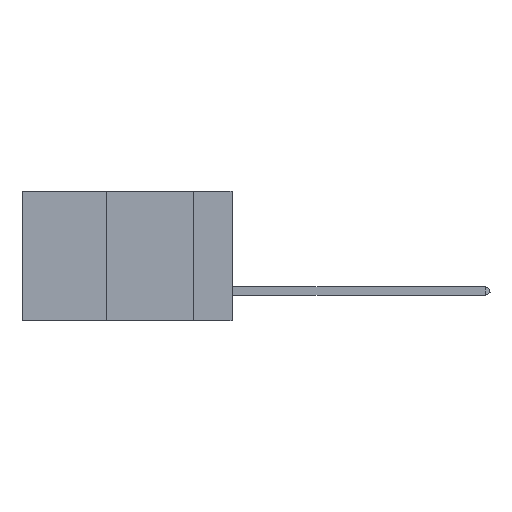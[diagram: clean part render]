
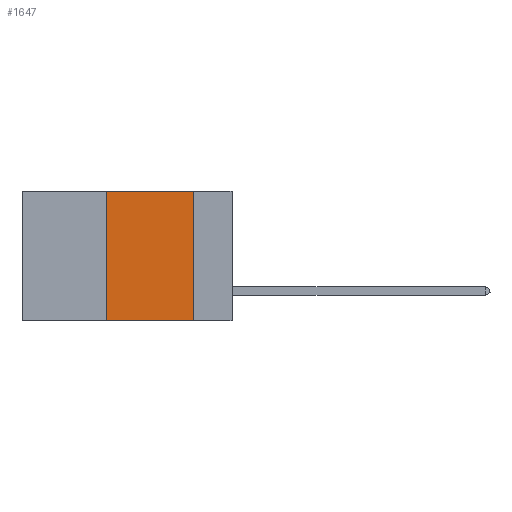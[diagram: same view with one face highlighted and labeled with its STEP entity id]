
A CAD part, left-side view. The second image highlights one B-rep face of the part: STEP entity #1647.
In plain terms, the highlighted planar face has unit normal (-1, 0, 0).
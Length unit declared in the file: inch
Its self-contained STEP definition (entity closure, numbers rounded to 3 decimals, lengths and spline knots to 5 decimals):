
#154 = AXIS2_PLACEMENT_3D ( 'NONE', #541, #16173, #9759 ) ;
#541 = CARTESIAN_POINT ( 'NONE',  ( 0., 0.6, 0. ) ) ;
#1647 = ADVANCED_FACE ( 'NONE', ( #8618 ), #12919, .F. ) ;
#1886 = LINE ( 'NONE', #2001, #4056 ) ;
#2001 = CARTESIAN_POINT ( 'NONE',  ( 0., 0.6, -0.37 ) ) ;
#2303 = EDGE_LOOP ( 'NONE', ( #15493, #11679, #3453, #10447 ) ) ;
#2762 = VECTOR ( 'NONE', #8040, 39.37008 ) ;
#3453 = ORIENTED_EDGE ( 'NONE', *, *, #18959, .F. ) ;
#4056 = VECTOR ( 'NONE', #7432, 39.37008 ) ;
#6481 = CARTESIAN_POINT ( 'NONE',  ( 0., 0.11, 0. ) ) ;
#7432 = DIRECTION ( 'NONE',  ( 0., -1., 0. ) ) ;
#7535 = CARTESIAN_POINT ( 'NONE',  ( 0., 0.36, 0. ) ) ;
#8040 = DIRECTION ( 'NONE',  ( 0., 0., -1. ) ) ;
#8618 = FACE_OUTER_BOUND ( 'NONE', #2303, .T. ) ;
#9755 = VECTOR ( 'NONE', #12947, 39.37008 ) ;
#9759 = DIRECTION ( 'NONE',  ( 0., 0., -1. ) ) ;
#9784 = CARTESIAN_POINT ( 'NONE',  ( 0., 0.36, 0. ) ) ;
#10231 = LINE ( 'NONE', #17434, #9755 ) ;
#10447 = ORIENTED_EDGE ( 'NONE', *, *, #11804, .T. ) ;
#10803 = VECTOR ( 'NONE', #12659, 39.37008 ) ;
#11021 = LINE ( 'NONE', #6481, #2762 ) ;
#11073 = LINE ( 'NONE', #9784, #10803 ) ;
#11168 = VERTEX_POINT ( 'NONE', #18367 ) ;
#11473 = VERTEX_POINT ( 'NONE', #11862 ) ;
#11511 = VERTEX_POINT ( 'NONE', #7535 ) ;
#11679 = ORIENTED_EDGE ( 'NONE', *, *, #16351, .F. ) ;
#11804 = EDGE_CURVE ( 'NONE', #16333, #11473, #1886, .T. ) ;
#11862 = CARTESIAN_POINT ( 'NONE',  ( 0., 0.11, -0.37 ) ) ;
#12659 = DIRECTION ( 'NONE',  ( 0., 0., 1. ) ) ;
#12877 = CARTESIAN_POINT ( 'NONE',  ( 0., 0.36, -0.37 ) ) ;
#12919 = PLANE ( 'NONE',  #154 ) ;
#12947 = DIRECTION ( 'NONE',  ( 0., -1., 0. ) ) ;
#14306 = EDGE_CURVE ( 'NONE', #11168, #11473, #11021, .T. ) ;
#15493 = ORIENTED_EDGE ( 'NONE', *, *, #14306, .F. ) ;
#16173 = DIRECTION ( 'NONE',  ( 1., 0., 0. ) ) ;
#16333 = VERTEX_POINT ( 'NONE', #12877 ) ;
#16351 = EDGE_CURVE ( 'NONE', #11511, #11168, #10231, .T. ) ;
#17434 = CARTESIAN_POINT ( 'NONE',  ( 0., 0.6, 0. ) ) ;
#18367 = CARTESIAN_POINT ( 'NONE',  ( 0., 0.11, 0. ) ) ;
#18959 = EDGE_CURVE ( 'NONE', #16333, #11511, #11073, .T. ) ;
